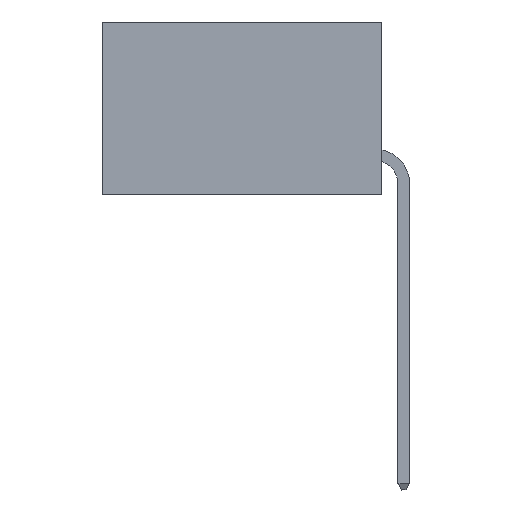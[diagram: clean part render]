
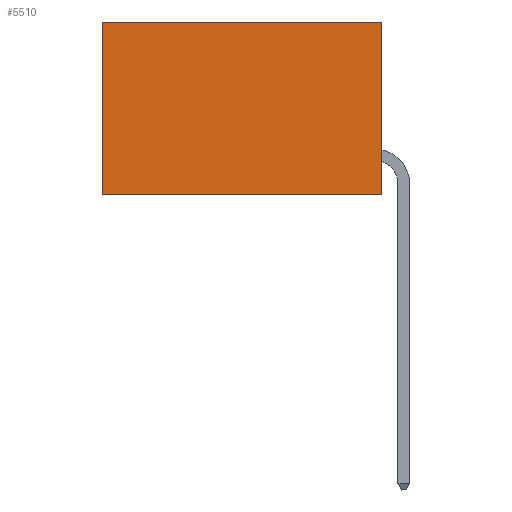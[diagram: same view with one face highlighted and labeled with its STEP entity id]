
A CAD part, left-side view. The second image highlights one B-rep face of the part: STEP entity #5510.
In plain terms, the highlighted planar face has unit normal (-1, 0, 0).
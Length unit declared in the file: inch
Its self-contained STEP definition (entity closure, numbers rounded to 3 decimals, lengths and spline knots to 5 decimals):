
#1277 = CARTESIAN_POINT ( 'NONE',  ( 0.2875, 0.6, -0.37 ) ) ;
#1933 = CARTESIAN_POINT ( 'NONE',  ( 0.2875, 0., 0. ) ) ;
#2584 = PLANE ( 'NONE',  #12180 ) ;
#2645 = EDGE_CURVE ( 'NONE', #12462, #6295, #9619, .T. ) ;
#2736 = CARTESIAN_POINT ( 'NONE',  ( 0.2875, 0.6, 0. ) ) ;
#3110 = DIRECTION ( 'NONE',  ( 0., 1., 0. ) ) ;
#3553 = VERTEX_POINT ( 'NONE', #1277 ) ;
#3965 = CARTESIAN_POINT ( 'NONE',  ( 0.2875, 0.6, 0. ) ) ;
#4284 = DIRECTION ( 'NONE',  ( 0., 1., 0. ) ) ;
#4735 = VECTOR ( 'NONE', #15025, 39.37008 ) ;
#5171 = EDGE_CURVE ( 'NONE', #12462, #15517, #12593, .T. ) ;
#5215 = ORIENTED_EDGE ( 'NONE', *, *, #5171, .T. ) ;
#5226 = VECTOR ( 'NONE', #3110, 39.37008 ) ;
#5510 = ADVANCED_FACE ( 'NONE', ( #10279 ), #2584, .F. ) ;
#5798 = CARTESIAN_POINT ( 'NONE',  ( 0.2875, 0., 0. ) ) ;
#6251 = ORIENTED_EDGE ( 'NONE', *, *, #15758, .F. ) ;
#6295 = VERTEX_POINT ( 'NONE', #7267 ) ;
#6477 = DIRECTION ( 'NONE',  ( 0., 0., -1. ) ) ;
#6504 = ORIENTED_EDGE ( 'NONE', *, *, #10392, .T. ) ;
#6998 = ORIENTED_EDGE ( 'NONE', *, *, #2645, .F. ) ;
#7267 = CARTESIAN_POINT ( 'NONE',  ( 0.2875, 0., -0.37 ) ) ;
#7460 = EDGE_LOOP ( 'NONE', ( #6504, #6251, #6998, #5215 ) ) ;
#7474 = DIRECTION ( 'NONE',  ( 0., 0., -1. ) ) ;
#7738 = CARTESIAN_POINT ( 'NONE',  ( 0.2875, 0., 0. ) ) ;
#8586 = CARTESIAN_POINT ( 'NONE',  ( 0.2875, 0., 0. ) ) ;
#9619 = LINE ( 'NONE', #7738, #4735 ) ;
#10279 = FACE_OUTER_BOUND ( 'NONE', #7460, .T. ) ;
#10392 = EDGE_CURVE ( 'NONE', #15517, #3553, #15588, .T. ) ;
#12180 = AXIS2_PLACEMENT_3D ( 'NONE', #8586, #15902, #7474 ) ;
#12462 = VERTEX_POINT ( 'NONE', #5798 ) ;
#12527 = LINE ( 'NONE', #15366, #13489 ) ;
#12593 = LINE ( 'NONE', #1933, #5226 ) ;
#13489 = VECTOR ( 'NONE', #4284, 39.37008 ) ;
#13665 = VECTOR ( 'NONE', #6477, 39.37008 ) ;
#15025 = DIRECTION ( 'NONE',  ( 0., 0., -1. ) ) ;
#15366 = CARTESIAN_POINT ( 'NONE',  ( 0.2875, 0., -0.37 ) ) ;
#15517 = VERTEX_POINT ( 'NONE', #3965 ) ;
#15588 = LINE ( 'NONE', #2736, #13665 ) ;
#15758 = EDGE_CURVE ( 'NONE', #6295, #3553, #12527, .T. ) ;
#15902 = DIRECTION ( 'NONE',  ( 1., 0., 0. ) ) ;
